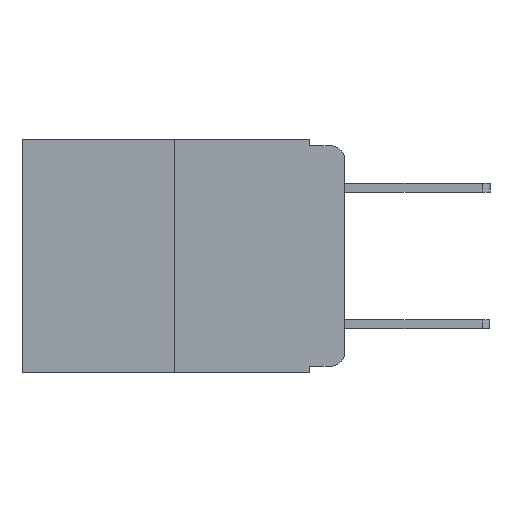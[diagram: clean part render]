
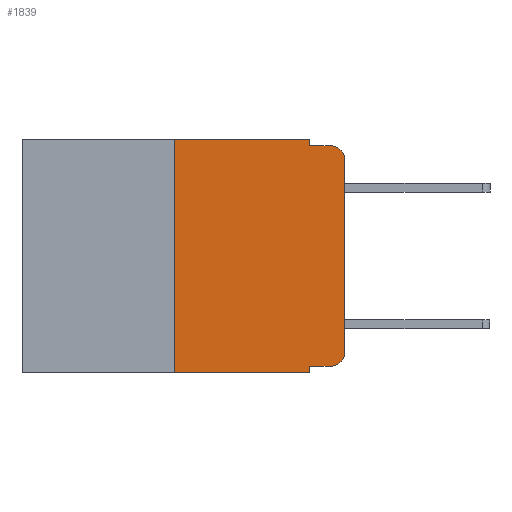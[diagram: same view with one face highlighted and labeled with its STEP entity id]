
A CAD part, left-side view. The second image highlights one B-rep face of the part: STEP entity #1839.
In plain terms, the highlighted planar face has unit normal (-1, 0, 0).
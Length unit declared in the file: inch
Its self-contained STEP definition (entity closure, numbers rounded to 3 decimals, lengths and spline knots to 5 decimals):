
#66 = DIRECTION ( 'NONE',  ( 0., 0., 1. ) ) ;
#223 = DIRECTION ( 'NONE',  ( 0., 0., -1. ) ) ;
#323 = DIRECTION ( 'NONE',  ( 0., 0., -1. ) ) ;
#552 = DIRECTION ( 'NONE',  ( -1., 0., 0. ) ) ;
#555 = CARTESIAN_POINT ( 'NONE',  ( 0., 0.02, -0.313 ) ) ;
#736 = CARTESIAN_POINT ( 'NONE',  ( 0., 0.25, -0.343 ) ) ;
#809 = CARTESIAN_POINT ( 'NONE',  ( 0., 0.051, -0.333 ) ) ;
#884 = EDGE_CURVE ( 'NONE', #2777, #3887, #1322, .T. ) ;
#1036 = VECTOR ( 'NONE', #66, 39.37008 ) ;
#1118 = VECTOR ( 'NONE', #7673, 39.37008 ) ;
#1120 = ORIENTED_EDGE ( 'NONE', *, *, #1912, .F. ) ;
#1174 = CARTESIAN_POINT ( 'NONE',  ( 0., 0., 0. ) ) ;
#1275 = EDGE_CURVE ( 'NONE', #3887, #5313, #2220, .T. ) ;
#1322 = LINE ( 'NONE', #3213, #1036 ) ;
#1436 = AXIS2_PLACEMENT_3D ( 'NONE', #6102, #5309, #4096 ) ;
#1753 = VERTEX_POINT ( 'NONE', #5728 ) ;
#1839 = ADVANCED_FACE ( 'NONE', ( #3765 ), #2159, .F. ) ;
#1887 = VERTEX_POINT ( 'NONE', #2058 ) ;
#1912 = EDGE_CURVE ( 'NONE', #3342, #6210, #9020, .T. ) ;
#2058 = CARTESIAN_POINT ( 'NONE',  ( 0., 0.02, -0.333 ) ) ;
#2087 = CARTESIAN_POINT ( 'NONE',  ( 0., 0.473, 0. ) ) ;
#2159 = PLANE ( 'NONE',  #7317 ) ;
#2220 = LINE ( 'NONE', #2087, #9418 ) ;
#2345 = DIRECTION ( 'NONE',  ( 0., -1., 0. ) ) ;
#2672 = DIRECTION ( 'NONE',  ( 0., 0., -1. ) ) ;
#2759 = VERTEX_POINT ( 'NONE', #7520 ) ;
#2777 = VERTEX_POINT ( 'NONE', #736 ) ;
#2814 = DIRECTION ( 'NONE',  ( 1., 0., 0. ) ) ;
#2818 = DIRECTION ( 'NONE',  ( 0., 0., 1. ) ) ;
#3077 = EDGE_CURVE ( 'NONE', #2777, #6210, #7222, .T. ) ;
#3148 = VECTOR ( 'NONE', #2818, 39.37008 ) ;
#3201 = CIRCLE ( 'NONE', #1436, 0.02 ) ;
#3213 = CARTESIAN_POINT ( 'NONE',  ( 0., 0.25, 0. ) ) ;
#3281 = CARTESIAN_POINT ( 'NONE',  ( 0., 0.473, 0. ) ) ;
#3342 = VERTEX_POINT ( 'NONE', #4933 ) ;
#3387 = VECTOR ( 'NONE', #7285, 39.37008 ) ;
#3467 = DIRECTION ( 'NONE',  ( 0., -1., 0. ) ) ;
#3483 = EDGE_CURVE ( 'NONE', #3342, #1887, #6945, .T. ) ;
#3735 = DIRECTION ( 'NONE',  ( 0., -1., 0. ) ) ;
#3765 = FACE_OUTER_BOUND ( 'NONE', #4791, .T. ) ;
#3887 = VERTEX_POINT ( 'NONE', #7553 ) ;
#4070 = LINE ( 'NONE', #4522, #9292 ) ;
#4096 = DIRECTION ( 'NONE',  ( 0., 0., -1. ) ) ;
#4181 = EDGE_CURVE ( 'NONE', #6761, #2759, #3201, .T. ) ;
#4522 = CARTESIAN_POINT ( 'NONE',  ( 0., 0.051, -0.01 ) ) ;
#4704 = CIRCLE ( 'NONE', #8119, 0.02 ) ;
#4791 = EDGE_LOOP ( 'NONE', ( #7924, #7997, #8251, #8140, #8530, #5678, #8351, #1120, #9248, #5805 ) ) ;
#4933 = CARTESIAN_POINT ( 'NONE',  ( 0., 0.051, -0.333 ) ) ;
#5078 = VECTOR ( 'NONE', #223, 39.37008 ) ;
#5309 = DIRECTION ( 'NONE',  ( -1., 0., 0. ) ) ;
#5313 = VERTEX_POINT ( 'NONE', #7210 ) ;
#5678 = ORIENTED_EDGE ( 'NONE', *, *, #884, .F. ) ;
#5720 = CARTESIAN_POINT ( 'NONE',  ( 0., 0.051, 0. ) ) ;
#5728 = CARTESIAN_POINT ( 'NONE',  ( 0., 0.051, -0.01 ) ) ;
#5805 = ORIENTED_EDGE ( 'NONE', *, *, #5996, .T. ) ;
#5996 = EDGE_CURVE ( 'NONE', #1887, #6234, #4704, .T. ) ;
#6102 = CARTESIAN_POINT ( 'NONE',  ( 0., 0.02, -0.03 ) ) ;
#6210 = VERTEX_POINT ( 'NONE', #7478 ) ;
#6234 = VERTEX_POINT ( 'NONE', #9223 ) ;
#6670 = EDGE_CURVE ( 'NONE', #6234, #6761, #8692, .T. ) ;
#6751 = VECTOR ( 'NONE', #3467, 39.37008 ) ;
#6761 = VERTEX_POINT ( 'NONE', #7037 ) ;
#6945 = LINE ( 'NONE', #809, #6751 ) ;
#7037 = CARTESIAN_POINT ( 'NONE',  ( 0., 0., -0.03 ) ) ;
#7210 = CARTESIAN_POINT ( 'NONE',  ( 0., 0.051, 0. ) ) ;
#7222 = LINE ( 'NONE', #7308, #3387 ) ;
#7225 = EDGE_CURVE ( 'NONE', #1753, #2759, #4070, .T. ) ;
#7285 = DIRECTION ( 'NONE',  ( 0., -1., 0. ) ) ;
#7308 = CARTESIAN_POINT ( 'NONE',  ( 0., 0.473, -0.343 ) ) ;
#7317 = AXIS2_PLACEMENT_3D ( 'NONE', #3281, #2814, #2672 ) ;
#7478 = CARTESIAN_POINT ( 'NONE',  ( 0., 0.051, -0.343 ) ) ;
#7489 = EDGE_CURVE ( 'NONE', #5313, #1753, #8597, .T. ) ;
#7520 = CARTESIAN_POINT ( 'NONE',  ( 0., 0.02, -0.01 ) ) ;
#7553 = CARTESIAN_POINT ( 'NONE',  ( 0., 0.25, 0. ) ) ;
#7673 = DIRECTION ( 'NONE',  ( 0., 0., -1. ) ) ;
#7924 = ORIENTED_EDGE ( 'NONE', *, *, #6670, .T. ) ;
#7997 = ORIENTED_EDGE ( 'NONE', *, *, #4181, .T. ) ;
#8119 = AXIS2_PLACEMENT_3D ( 'NONE', #555, #552, #323 ) ;
#8140 = ORIENTED_EDGE ( 'NONE', *, *, #7489, .F. ) ;
#8251 = ORIENTED_EDGE ( 'NONE', *, *, #7225, .F. ) ;
#8316 = CARTESIAN_POINT ( 'NONE',  ( 0., 0.051, 0. ) ) ;
#8351 = ORIENTED_EDGE ( 'NONE', *, *, #3077, .T. ) ;
#8530 = ORIENTED_EDGE ( 'NONE', *, *, #1275, .F. ) ;
#8597 = LINE ( 'NONE', #8316, #1118 ) ;
#8692 = LINE ( 'NONE', #1174, #3148 ) ;
#9020 = LINE ( 'NONE', #5720, #5078 ) ;
#9223 = CARTESIAN_POINT ( 'NONE',  ( 0., 0., -0.313 ) ) ;
#9248 = ORIENTED_EDGE ( 'NONE', *, *, #3483, .T. ) ;
#9292 = VECTOR ( 'NONE', #3735, 39.37008 ) ;
#9418 = VECTOR ( 'NONE', #2345, 39.37008 ) ;
